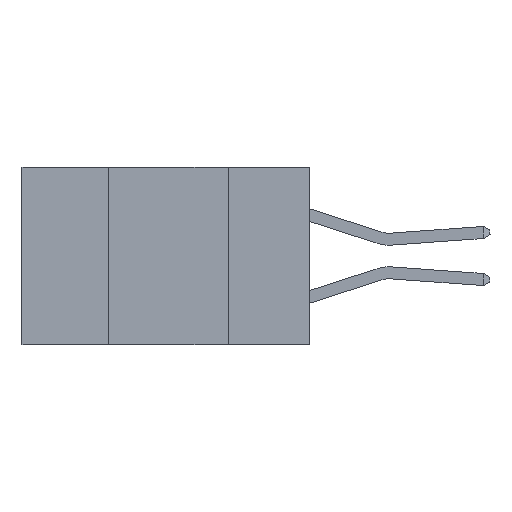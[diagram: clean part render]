
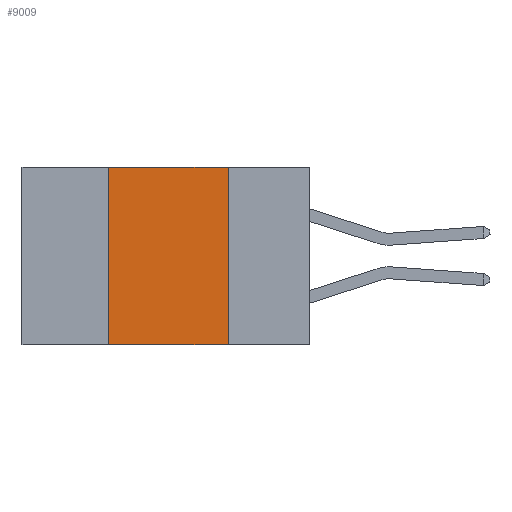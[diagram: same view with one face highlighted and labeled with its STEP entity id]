
A CAD part, left-side view. The second image highlights one B-rep face of the part: STEP entity #9009.
In plain terms, the highlighted planar face has unit normal (-1, 0, 0).
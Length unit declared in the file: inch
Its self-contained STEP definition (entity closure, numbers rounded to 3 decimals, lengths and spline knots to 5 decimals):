
#856 = LINE ( 'NONE', #14380, #13026 ) ;
#1652 = VERTEX_POINT ( 'NONE', #10283 ) ;
#2123 = DIRECTION ( 'NONE',  ( 0., 0., -1. ) ) ;
#2460 = DIRECTION ( 'NONE',  ( 1., 0., 0. ) ) ;
#2635 = DIRECTION ( 'NONE',  ( 0., 0., 1. ) ) ;
#2672 = VERTEX_POINT ( 'NONE', #16754 ) ;
#4042 = CARTESIAN_POINT ( 'NONE',  ( 0., 0.6, 0. ) ) ;
#4437 = LINE ( 'NONE', #14895, #13686 ) ;
#4751 = CARTESIAN_POINT ( 'NONE',  ( 0., 0.6, 0. ) ) ;
#5710 = DIRECTION ( 'NONE',  ( 0., 0., -1. ) ) ;
#5767 = LINE ( 'NONE', #21119, #11861 ) ;
#6284 = EDGE_CURVE ( 'NONE', #17206, #2672, #4437, .T. ) ;
#7023 = ORIENTED_EDGE ( 'NONE', *, *, #11369, .T. ) ;
#7565 = VERTEX_POINT ( 'NONE', #19383 ) ;
#9009 = ADVANCED_FACE ( 'NONE', ( #19699 ), #16078, .F. ) ;
#9367 = DIRECTION ( 'NONE',  ( 0., -1., 0. ) ) ;
#9955 = ORIENTED_EDGE ( 'NONE', *, *, #16044, .F. ) ;
#10283 = CARTESIAN_POINT ( 'NONE',  ( 0., 0.17, -0.37 ) ) ;
#10701 = AXIS2_PLACEMENT_3D ( 'NONE', #4042, #2460, #5710 ) ;
#11369 = EDGE_CURVE ( 'NONE', #17206, #1652, #5767, .T. ) ;
#11637 = VECTOR ( 'NONE', #9367, 39.37008 ) ;
#11861 = VECTOR ( 'NONE', #21013, 39.37008 ) ;
#13026 = VECTOR ( 'NONE', #2123, 39.37008 ) ;
#13686 = VECTOR ( 'NONE', #2635, 39.37008 ) ;
#13806 = EDGE_CURVE ( 'NONE', #7565, #1652, #856, .T. ) ;
#13829 = ORIENTED_EDGE ( 'NONE', *, *, #6284, .F. ) ;
#14380 = CARTESIAN_POINT ( 'NONE',  ( 0., 0.17, -0.37 ) ) ;
#14895 = CARTESIAN_POINT ( 'NONE',  ( 0., 0.42, -0.37 ) ) ;
#16044 = EDGE_CURVE ( 'NONE', #2672, #7565, #16481, .T. ) ;
#16049 = ORIENTED_EDGE ( 'NONE', *, *, #13806, .F. ) ;
#16078 = PLANE ( 'NONE',  #10701 ) ;
#16481 = LINE ( 'NONE', #4751, #11637 ) ;
#16754 = CARTESIAN_POINT ( 'NONE',  ( 0., 0.42, 0. ) ) ;
#17206 = VERTEX_POINT ( 'NONE', #20910 ) ;
#18542 = EDGE_LOOP ( 'NONE', ( #16049, #9955, #13829, #7023 ) ) ;
#19383 = CARTESIAN_POINT ( 'NONE',  ( 0., 0.17, 0. ) ) ;
#19699 = FACE_OUTER_BOUND ( 'NONE', #18542, .T. ) ;
#20910 = CARTESIAN_POINT ( 'NONE',  ( 0., 0.42, -0.37 ) ) ;
#21013 = DIRECTION ( 'NONE',  ( 0., -1., 0. ) ) ;
#21119 = CARTESIAN_POINT ( 'NONE',  ( 0., 0.6, -0.37 ) ) ;
